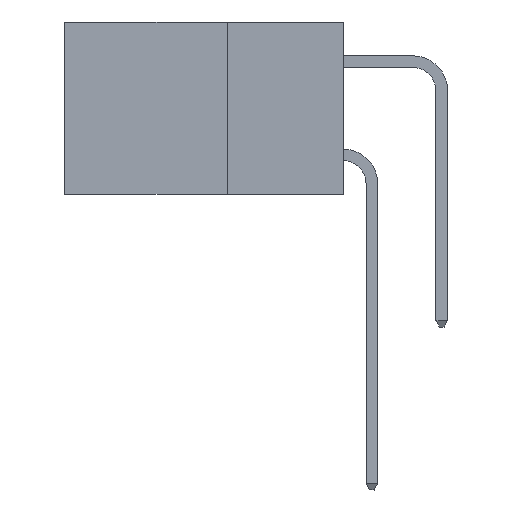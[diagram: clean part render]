
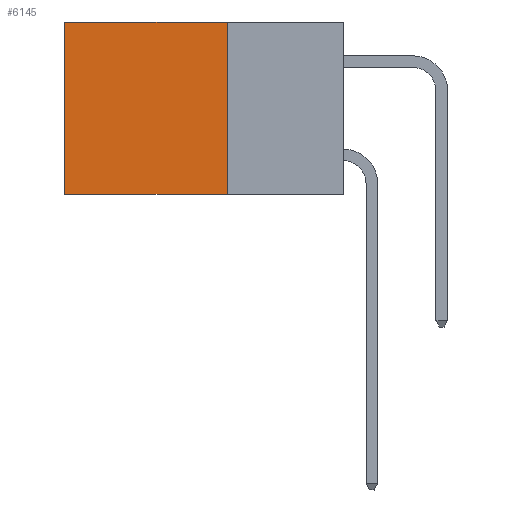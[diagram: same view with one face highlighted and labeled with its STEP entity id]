
A CAD part, left-side view. The second image highlights one B-rep face of the part: STEP entity #6145.
In plain terms, the highlighted planar face has unit normal (-1, 0, 0).
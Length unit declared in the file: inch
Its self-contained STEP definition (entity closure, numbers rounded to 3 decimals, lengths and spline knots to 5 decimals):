
#1910 = DIRECTION ( 'NONE',  ( 1., 0., 0. ) ) ;
#2500 = DIRECTION ( 'NONE',  ( 0., 1., 0. ) ) ;
#3010 = EDGE_CURVE ( 'NONE', #22590, #17052, #13390, .T. ) ;
#3207 = ORIENTED_EDGE ( 'NONE', *, *, #3010, .F. ) ;
#3448 = FACE_OUTER_BOUND ( 'NONE', #20672, .T. ) ;
#3704 = VECTOR ( 'NONE', #11239, 39.37008 ) ;
#3817 = DIRECTION ( 'NONE',  ( 0., 0., -1. ) ) ;
#5500 = DIRECTION ( 'NONE',  ( 0., 0., -1. ) ) ;
#5747 = VERTEX_POINT ( 'NONE', #21534 ) ;
#6145 = ADVANCED_FACE ( 'NONE', ( #3448 ), #14113, .F. ) ;
#7369 = LINE ( 'NONE', #14425, #19802 ) ;
#7711 = CARTESIAN_POINT ( 'NONE',  ( 0.2615, 0.25, 0. ) ) ;
#8671 = ORIENTED_EDGE ( 'NONE', *, *, #16713, .T. ) ;
#9168 = CARTESIAN_POINT ( 'NONE',  ( 0.2615, 0.25, -0.37 ) ) ;
#9779 = AXIS2_PLACEMENT_3D ( 'NONE', #9168, #1910, #19861 ) ;
#9806 = EDGE_CURVE ( 'NONE', #5747, #22590, #16474, .T. ) ;
#11239 = DIRECTION ( 'NONE',  ( 0., 1., 0. ) ) ;
#11409 = CARTESIAN_POINT ( 'NONE',  ( 0.2615, 0.25, -0.37 ) ) ;
#11758 = VECTOR ( 'NONE', #2500, 39.37008 ) ;
#13331 = ORIENTED_EDGE ( 'NONE', *, *, #16783, .T. ) ;
#13390 = LINE ( 'NONE', #11409, #11758 ) ;
#14113 = PLANE ( 'NONE',  #9779 ) ;
#14425 = CARTESIAN_POINT ( 'NONE',  ( 0.2615, 0.6, -0.37 ) ) ;
#15381 = ORIENTED_EDGE ( 'NONE', *, *, #9806, .F. ) ;
#16158 = CARTESIAN_POINT ( 'NONE',  ( 0.2615, 0.25, -0.37 ) ) ;
#16474 = LINE ( 'NONE', #17695, #20718 ) ;
#16713 = EDGE_CURVE ( 'NONE', #18086, #17052, #7369, .T. ) ;
#16783 = EDGE_CURVE ( 'NONE', #5747, #18086, #20062, .T. ) ;
#17052 = VERTEX_POINT ( 'NONE', #22987 ) ;
#17695 = CARTESIAN_POINT ( 'NONE',  ( 0.2615, 0.25, -0.37 ) ) ;
#18086 = VERTEX_POINT ( 'NONE', #18265 ) ;
#18265 = CARTESIAN_POINT ( 'NONE',  ( 0.2615, 0.6, 0. ) ) ;
#19802 = VECTOR ( 'NONE', #5500, 39.37008 ) ;
#19861 = DIRECTION ( 'NONE',  ( 0., 0., -1. ) ) ;
#20062 = LINE ( 'NONE', #7711, #3704 ) ;
#20672 = EDGE_LOOP ( 'NONE', ( #8671, #3207, #15381, #13331 ) ) ;
#20718 = VECTOR ( 'NONE', #3817, 39.37008 ) ;
#21534 = CARTESIAN_POINT ( 'NONE',  ( 0.2615, 0.25, 0. ) ) ;
#22590 = VERTEX_POINT ( 'NONE', #16158 ) ;
#22987 = CARTESIAN_POINT ( 'NONE',  ( 0.2615, 0.6, -0.37 ) ) ;
